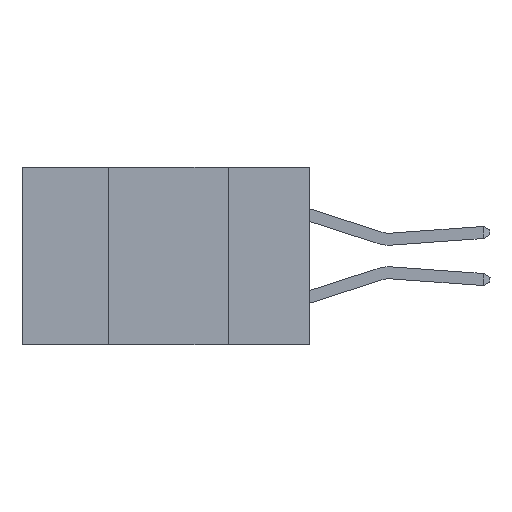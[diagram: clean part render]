
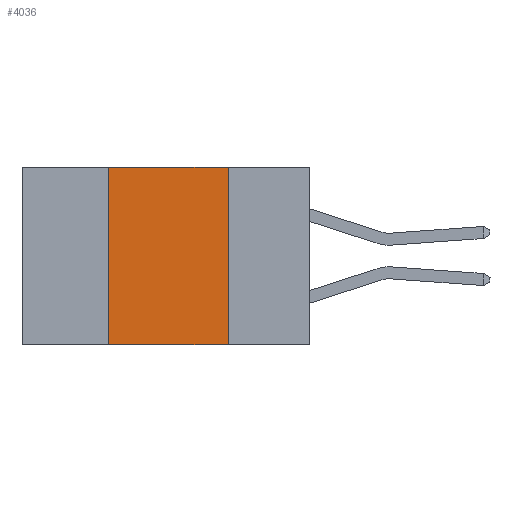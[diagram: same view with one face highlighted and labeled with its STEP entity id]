
A CAD part, left-side view. The second image highlights one B-rep face of the part: STEP entity #4036.
In plain terms, the highlighted planar face has unit normal (-1, 0, 0).
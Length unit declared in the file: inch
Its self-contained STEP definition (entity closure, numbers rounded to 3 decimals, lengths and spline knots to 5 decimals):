
#1021 = DIRECTION ( 'NONE',  ( 0., -1., 0. ) ) ;
#1054 = CARTESIAN_POINT ( 'NONE',  ( 0., 0.17, 0. ) ) ;
#1464 = VECTOR ( 'NONE', #1021, 39.37008 ) ;
#1506 = CARTESIAN_POINT ( 'NONE',  ( 0., 0.17, -0.37 ) ) ;
#1566 = LINE ( 'NONE', #1054, #9922 ) ;
#1733 = DIRECTION ( 'NONE',  ( 0., 0., -1. ) ) ;
#1942 = EDGE_CURVE ( 'NONE', #12008, #8956, #2704, .T. ) ;
#2704 = LINE ( 'NONE', #3182, #1464 ) ;
#2905 = VERTEX_POINT ( 'NONE', #1506 ) ;
#3182 = CARTESIAN_POINT ( 'NONE',  ( 0., 0.6, 0. ) ) ;
#3339 = ORIENTED_EDGE ( 'NONE', *, *, #3535, .F. ) ;
#3535 = EDGE_CURVE ( 'NONE', #8956, #2905, #1566, .T. ) ;
#3845 = FACE_OUTER_BOUND ( 'NONE', #11864, .T. ) ;
#4036 = ADVANCED_FACE ( 'NONE', ( #3845 ), #9196, .F. ) ;
#4164 = DIRECTION ( 'NONE',  ( 1., 0., 0. ) ) ;
#4487 = DIRECTION ( 'NONE',  ( 0., -1., 0. ) ) ;
#4910 = EDGE_CURVE ( 'NONE', #6586, #12008, #10489, .T. ) ;
#4920 = CARTESIAN_POINT ( 'NONE',  ( 0., 0.42, 0. ) ) ;
#4942 = CARTESIAN_POINT ( 'NONE',  ( 0., 0.42, 0. ) ) ;
#5116 = ORIENTED_EDGE ( 'NONE', *, *, #12564, .T. ) ;
#6586 = VERTEX_POINT ( 'NONE', #12630 ) ;
#7046 = AXIS2_PLACEMENT_3D ( 'NONE', #11135, #4164, #10193 ) ;
#7636 = ORIENTED_EDGE ( 'NONE', *, *, #4910, .F. ) ;
#7768 = DIRECTION ( 'NONE',  ( 0., 0., 1. ) ) ;
#7860 = VECTOR ( 'NONE', #7768, 39.37008 ) ;
#8119 = ORIENTED_EDGE ( 'NONE', *, *, #1942, .F. ) ;
#8956 = VERTEX_POINT ( 'NONE', #10590 ) ;
#9196 = PLANE ( 'NONE',  #7046 ) ;
#9922 = VECTOR ( 'NONE', #1733, 39.37008 ) ;
#10025 = VECTOR ( 'NONE', #4487, 39.37008 ) ;
#10193 = DIRECTION ( 'NONE',  ( 0., 0., -1. ) ) ;
#10410 = CARTESIAN_POINT ( 'NONE',  ( 0., 0.6, -0.37 ) ) ;
#10489 = LINE ( 'NONE', #4920, #7860 ) ;
#10590 = CARTESIAN_POINT ( 'NONE',  ( 0., 0.17, 0. ) ) ;
#10781 = LINE ( 'NONE', #10410, #10025 ) ;
#11135 = CARTESIAN_POINT ( 'NONE',  ( 0., 0.6, 0. ) ) ;
#11864 = EDGE_LOOP ( 'NONE', ( #3339, #8119, #7636, #5116 ) ) ;
#12008 = VERTEX_POINT ( 'NONE', #4942 ) ;
#12564 = EDGE_CURVE ( 'NONE', #6586, #2905, #10781, .T. ) ;
#12630 = CARTESIAN_POINT ( 'NONE',  ( 0., 0.42, -0.37 ) ) ;
